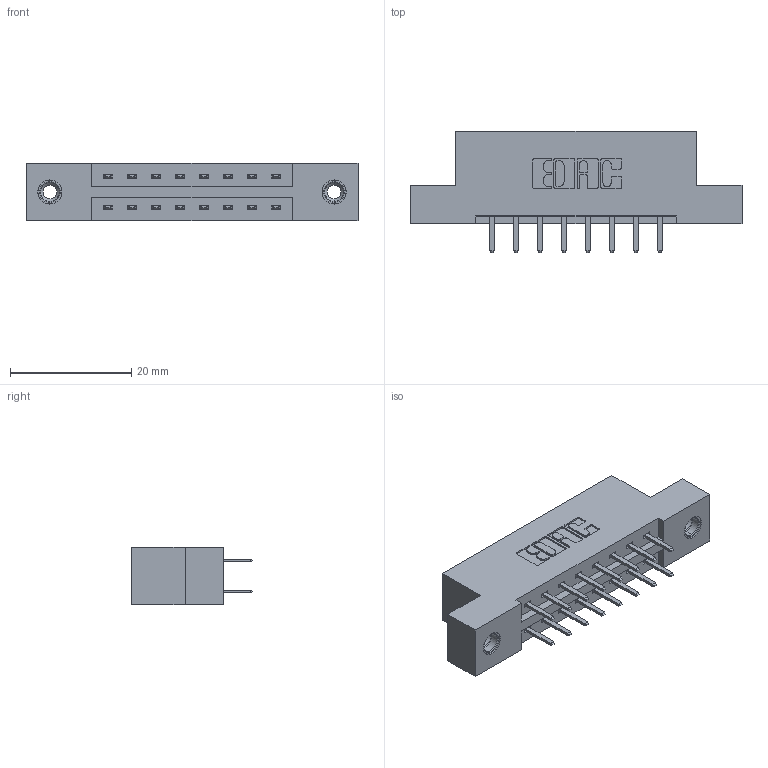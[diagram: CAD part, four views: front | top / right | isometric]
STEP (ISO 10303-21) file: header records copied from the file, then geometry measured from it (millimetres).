
FILE_DESCRIPTION (( 'STEP AP203' ), '1' );
FILE_NAME ('387-016-520-208.STEP', '2019-10-15T22:29:06', ( '' ), ( '' ), 'SwSTEP 2.0', 'SolidWorks 2016', '' );
FILE_SCHEMA (( 'CONFIG_CONTROL_DESIGN' ));
Length unit declared in the file: inch
Products named in the file (4): 345-292-001_345-293-120; 337 Part_Flush Mounting Lugs - 0.156 Dia-TI; 345-250-001_345-250-003-102; 387-016-520-208
Assembly tree (19 placements, depth 2):
  387-016-520-208
    337 Part_Flush Mounting Lugs - 0.156 Dia-TI
    345-292-001_345-293-120  x16
    345-250-001_345-250-003-102  x2
Bounding box: 54.71 x 20.02 x 9.4 mm (x, y, z)
Volume: 5299.8 mm3; surface area: 5665.1 mm2
Topology: 19 solids, 19 shells, 1102 faces, 3151 edges, 2050 vertices
Faces by surface type: plane 742, cylinder 344, cone 12, torus 4
Entity records: 11900 total; most frequent: CARTESIAN_POINT 2025, ORIENTED_EDGE 1942, DIRECTION 1805, EDGE_CURVE 971, VECTOR 819, LINE 819, VERTEX_POINT 640, AXIS2_PLACEMENT_3D 493
